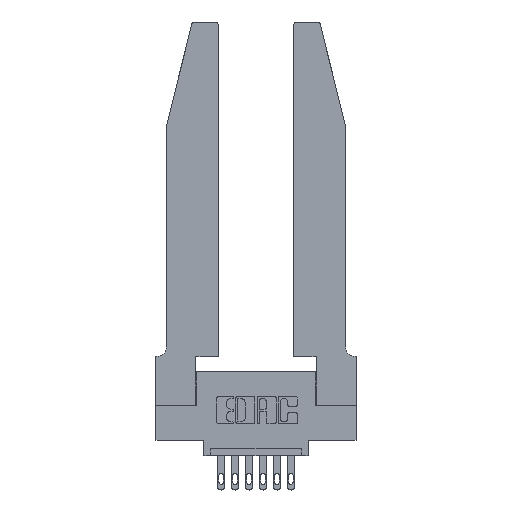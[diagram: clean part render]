
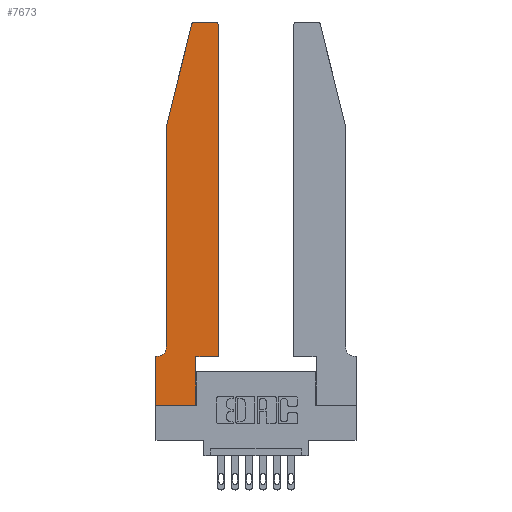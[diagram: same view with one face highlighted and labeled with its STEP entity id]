
A CAD part, top view. The second image highlights one B-rep face of the part: STEP entity #7673.
In plain terms, the highlighted planar face has unit normal (0, 0, 1).
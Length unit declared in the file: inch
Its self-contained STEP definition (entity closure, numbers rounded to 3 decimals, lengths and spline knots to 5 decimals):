
#235 = EDGE_CURVE ( 'NONE', #1704, #1128, #1821, .T. ) ;
#487 = LINE ( 'NONE', #11788, #12487 ) ;
#776 = VECTOR ( 'NONE', #10958, 39.37008 ) ;
#986 = ORIENTED_EDGE ( 'NONE', *, *, #9761, .T. ) ;
#1043 = FACE_OUTER_BOUND ( 'NONE', #5464, .T. ) ;
#1092 = DIRECTION ( 'NONE',  ( 0., -1., 0. ) ) ;
#1128 = VERTEX_POINT ( 'NONE', #10629 ) ;
#1359 = CARTESIAN_POINT ( 'NONE',  ( 0.0055, 0.42, 0.37 ) ) ;
#1552 = CARTESIAN_POINT ( 'NONE',  ( 0.4505, 0.35, 0.37 ) ) ;
#1648 = DIRECTION ( 'NONE',  ( 0., -1., 0. ) ) ;
#1683 = CIRCLE ( 'NONE', #2147, 0.03 ) ;
#1704 = VERTEX_POINT ( 'NONE', #1552 ) ;
#1821 = LINE ( 'NONE', #9156, #10226 ) ;
#1865 = EDGE_CURVE ( 'NONE', #10797, #1704, #10034, .T. ) ;
#1869 = LINE ( 'NONE', #3894, #5287 ) ;
#1916 = VECTOR ( 'NONE', #8946, 39.37008 ) ;
#1949 = VERTEX_POINT ( 'NONE', #3116 ) ;
#1965 = AXIS2_PLACEMENT_3D ( 'NONE', #11152, #9996, #13420 ) ;
#2147 = AXIS2_PLACEMENT_3D ( 'NONE', #11208, #12381, #3679 ) ;
#2373 = AXIS2_PLACEMENT_3D ( 'NONE', #1359, #10112, #10450 ) ;
#2378 = PLANE ( 'NONE',  #1965 ) ;
#2455 = CARTESIAN_POINT ( 'NONE',  ( 0.0055, 0.35, 0.37 ) ) ;
#3093 = EDGE_CURVE ( 'NONE', #13960, #7020, #8608, .T. ) ;
#3116 = CARTESIAN_POINT ( 'NONE',  ( 0.0755, 0.42, 0.37 ) ) ;
#3416 = CARTESIAN_POINT ( 'NONE',  ( 0.2865, 0.35, 0.37 ) ) ;
#3565 = EDGE_CURVE ( 'NONE', #8252, #6105, #6212, .T. ) ;
#3596 = DIRECTION ( 'NONE',  ( 0., 1., 0. ) ) ;
#3679 = DIRECTION ( 'NONE',  ( 1., 0., 0. ) ) ;
#3698 = EDGE_CURVE ( 'NONE', #1128, #8252, #6721, .T. ) ;
#3894 = CARTESIAN_POINT ( 'NONE',  ( 0.0755, 2., 0.37 ) ) ;
#3966 = CARTESIAN_POINT ( 'NONE',  ( 0.284, 2.75, 0.37 ) ) ;
#4676 = ORIENTED_EDGE ( 'NONE', *, *, #235, .T. ) ;
#4873 = EDGE_CURVE ( 'NONE', #7020, #5873, #7696, .T. ) ;
#5177 = VECTOR ( 'NONE', #12242, 39.37008 ) ;
#5255 = EDGE_CURVE ( 'NONE', #12367, #1949, #1869, .T. ) ;
#5287 = VECTOR ( 'NONE', #1648, 39.37008 ) ;
#5464 = EDGE_LOOP ( 'NONE', ( #6038, #5517, #986, #8002, #11507, #8814, #8622, #12657, #10759, #13978, #4676, #9551 ) ) ;
#5517 = ORIENTED_EDGE ( 'NONE', *, *, #8482, .T. ) ;
#5621 = DIRECTION ( 'NONE',  ( 1., 0., 0. ) ) ;
#5873 = VERTEX_POINT ( 'NONE', #9387 ) ;
#6038 = ORIENTED_EDGE ( 'NONE', *, *, #3565, .T. ) ;
#6074 = CARTESIAN_POINT ( 'NONE',  ( 0.25487, 2.72718, 0.37 ) ) ;
#6105 = VERTEX_POINT ( 'NONE', #3966 ) ;
#6212 = LINE ( 'NONE', #8996, #1916 ) ;
#6537 = VERTEX_POINT ( 'NONE', #6074 ) ;
#6634 = CARTESIAN_POINT ( 'NONE',  ( 0., 0., 0.37 ) ) ;
#6683 = VECTOR ( 'NONE', #1092, 39.37008 ) ;
#6721 = CIRCLE ( 'NONE', #7076, 0.03 ) ;
#6925 = LINE ( 'NONE', #3416, #776 ) ;
#7020 = VERTEX_POINT ( 'NONE', #11574 ) ;
#7052 = CARTESIAN_POINT ( 'NONE',  ( 0.2865, 0.35, 0.37 ) ) ;
#7076 = AXIS2_PLACEMENT_3D ( 'NONE', #12665, #8029, #12615 ) ;
#7126 = VECTOR ( 'NONE', #8765, 39.37008 ) ;
#7460 = CARTESIAN_POINT ( 'NONE',  ( 0.4205, 2.75, 0.37 ) ) ;
#7673 = ADVANCED_FACE ( 'NONE', ( #1043 ), #2378, .T. ) ;
#7696 = LINE ( 'NONE', #6634, #6683 ) ;
#7830 = CARTESIAN_POINT ( 'NONE',  ( 0.2865, 0., 0.37 ) ) ;
#8002 = ORIENTED_EDGE ( 'NONE', *, *, #5255, .T. ) ;
#8029 = DIRECTION ( 'NONE',  ( 0., 0., 1. ) ) ;
#8252 = VERTEX_POINT ( 'NONE', #7460 ) ;
#8482 = EDGE_CURVE ( 'NONE', #6105, #6537, #1683, .T. ) ;
#8571 = LINE ( 'NONE', #9998, #13752 ) ;
#8608 = LINE ( 'NONE', #12851, #5177 ) ;
#8622 = ORIENTED_EDGE ( 'NONE', *, *, #4873, .T. ) ;
#8765 = DIRECTION ( 'NONE',  ( 1., 0., 0. ) ) ;
#8814 = ORIENTED_EDGE ( 'NONE', *, *, #3093, .T. ) ;
#8946 = DIRECTION ( 'NONE',  ( -1., 0., 0. ) ) ;
#8996 = CARTESIAN_POINT ( 'NONE',  ( 0.2605, 2.75, 0.37 ) ) ;
#9156 = CARTESIAN_POINT ( 'NONE',  ( 0.4505, 0.35, 0.37 ) ) ;
#9387 = CARTESIAN_POINT ( 'NONE',  ( 0., 0., 0.37 ) ) ;
#9405 = VERTEX_POINT ( 'NONE', #7830 ) ;
#9551 = ORIENTED_EDGE ( 'NONE', *, *, #3698, .T. ) ;
#9761 = EDGE_CURVE ( 'NONE', #6537, #12367, #487, .T. ) ;
#9996 = DIRECTION ( 'NONE',  ( 0., 0., 1. ) ) ;
#9998 = CARTESIAN_POINT ( 'NONE',  ( 0., 0., 0.37 ) ) ;
#10034 = LINE ( 'NONE', #13158, #7126 ) ;
#10112 = DIRECTION ( 'NONE',  ( 0., 0., -1. ) ) ;
#10226 = VECTOR ( 'NONE', #3596, 39.37008 ) ;
#10450 = DIRECTION ( 'NONE',  ( -1., 0., 0. ) ) ;
#10629 = CARTESIAN_POINT ( 'NONE',  ( 0.4505, 2.72, 0.37 ) ) ;
#10759 = ORIENTED_EDGE ( 'NONE', *, *, #11186, .T. ) ;
#10797 = VERTEX_POINT ( 'NONE', #7052 ) ;
#10958 = DIRECTION ( 'NONE',  ( 0., 1., 0. ) ) ;
#11152 = CARTESIAN_POINT ( 'NONE',  ( 0., 0.35, 0.37 ) ) ;
#11186 = EDGE_CURVE ( 'NONE', #9405, #10797, #6925, .T. ) ;
#11208 = CARTESIAN_POINT ( 'NONE',  ( 0.284, 2.72, 0.37 ) ) ;
#11448 = CIRCLE ( 'NONE', #2373, 0.07 ) ;
#11507 = ORIENTED_EDGE ( 'NONE', *, *, #14025, .T. ) ;
#11574 = CARTESIAN_POINT ( 'NONE',  ( 0., 0.35, 0.37 ) ) ;
#11788 = CARTESIAN_POINT ( 'NONE',  ( 0.0755, 2., 0.37 ) ) ;
#11834 = DIRECTION ( 'NONE',  ( -0.239, -0.971, 0. ) ) ;
#12242 = DIRECTION ( 'NONE',  ( -1., 0., 0. ) ) ;
#12367 = VERTEX_POINT ( 'NONE', #12825 ) ;
#12381 = DIRECTION ( 'NONE',  ( 0., 0., 1. ) ) ;
#12487 = VECTOR ( 'NONE', #11834, 39.37008 ) ;
#12615 = DIRECTION ( 'NONE',  ( 1., 0., 0. ) ) ;
#12657 = ORIENTED_EDGE ( 'NONE', *, *, #12764, .T. ) ;
#12665 = CARTESIAN_POINT ( 'NONE',  ( 0.4205, 2.72, 0.37 ) ) ;
#12764 = EDGE_CURVE ( 'NONE', #5873, #9405, #8571, .T. ) ;
#12825 = CARTESIAN_POINT ( 'NONE',  ( 0.0755, 2., 0.37 ) ) ;
#12851 = CARTESIAN_POINT ( 'NONE',  ( 0.0755, 0.35, 0.37 ) ) ;
#13158 = CARTESIAN_POINT ( 'NONE',  ( 0.4505, 0.35, 0.37 ) ) ;
#13420 = DIRECTION ( 'NONE',  ( 1., 0., 0. ) ) ;
#13752 = VECTOR ( 'NONE', #5621, 39.37008 ) ;
#13960 = VERTEX_POINT ( 'NONE', #2455 ) ;
#13978 = ORIENTED_EDGE ( 'NONE', *, *, #1865, .T. ) ;
#14025 = EDGE_CURVE ( 'NONE', #1949, #13960, #11448, .T. ) ;
